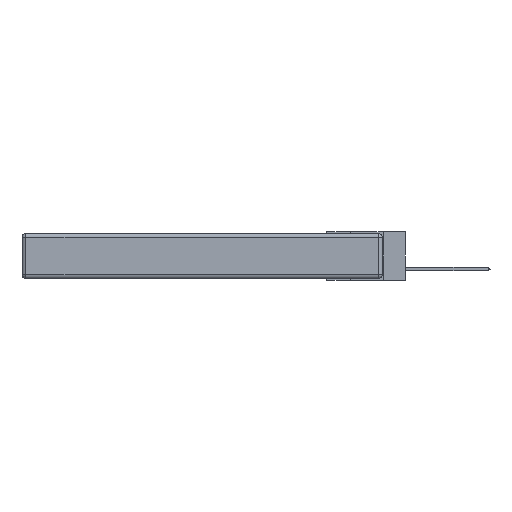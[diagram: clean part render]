
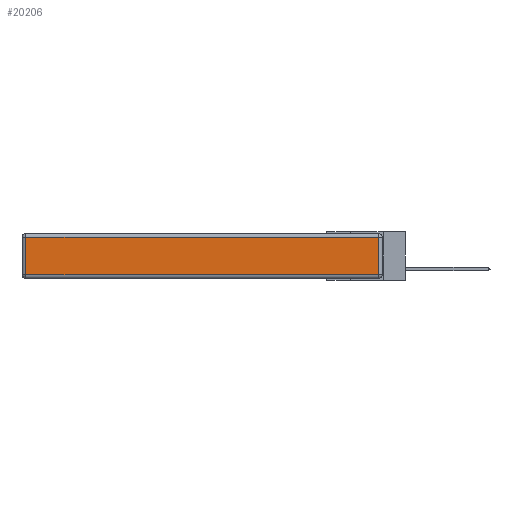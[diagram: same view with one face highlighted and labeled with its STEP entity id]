
A CAD part, left-side view. The second image highlights one B-rep face of the part: STEP entity #20206.
In plain terms, the highlighted planar face has unit normal (-1, 0, 0).
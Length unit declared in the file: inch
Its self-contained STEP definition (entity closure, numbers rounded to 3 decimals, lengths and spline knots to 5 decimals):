
#370 = VERTEX_POINT ( 'NONE', #17069 ) ;
#1235 = VECTOR ( 'NONE', #6113, 39.37008 ) ;
#2106 = VECTOR ( 'NONE', #9642, 39.37008 ) ;
#2582 = DIRECTION ( 'NONE',  ( 0., 0., -1. ) ) ;
#3070 = LINE ( 'NONE', #13655, #12551 ) ;
#6113 = DIRECTION ( 'NONE',  ( 0., 1., 0. ) ) ;
#6218 = EDGE_CURVE ( 'NONE', #370, #7089, #12154, .T. ) ;
#6316 = EDGE_CURVE ( 'NONE', #11339, #370, #19280, .T. ) ;
#6589 = ORIENTED_EDGE ( 'NONE', *, *, #10112, .T. ) ;
#7089 = VERTEX_POINT ( 'NONE', #19322 ) ;
#7811 = CARTESIAN_POINT ( 'NONE',  ( 0., 0.03, -0.343 ) ) ;
#8239 = VERTEX_POINT ( 'NONE', #21363 ) ;
#8573 = ORIENTED_EDGE ( 'NONE', *, *, #6218, .T. ) ;
#9642 = DIRECTION ( 'NONE',  ( 0., -1., 0. ) ) ;
#10112 = EDGE_CURVE ( 'NONE', #7089, #8239, #3070, .T. ) ;
#10745 = EDGE_CURVE ( 'NONE', #8239, #11339, #16156, .T. ) ;
#11339 = VERTEX_POINT ( 'NONE', #16797 ) ;
#11416 = EDGE_LOOP ( 'NONE', ( #15464, #17582, #8573, #6589 ) ) ;
#11490 = DIRECTION ( 'NONE',  ( 0., 0., 1. ) ) ;
#11632 = CARTESIAN_POINT ( 'NONE',  ( 0., 0., -0.313 ) ) ;
#12154 = LINE ( 'NONE', #18725, #1235 ) ;
#12551 = VECTOR ( 'NONE', #2582, 39.37008 ) ;
#13244 = AXIS2_PLACEMENT_3D ( 'NONE', #15725, #20925, #19308 ) ;
#13655 = CARTESIAN_POINT ( 'NONE',  ( 0., 2.72, -0.343 ) ) ;
#15464 = ORIENTED_EDGE ( 'NONE', *, *, #10745, .T. ) ;
#15725 = CARTESIAN_POINT ( 'NONE',  ( 0., 0., -0.343 ) ) ;
#16156 = LINE ( 'NONE', #11632, #2106 ) ;
#16785 = FACE_OUTER_BOUND ( 'NONE', #11416, .T. ) ;
#16797 = CARTESIAN_POINT ( 'NONE',  ( 0., 0.03, -0.313 ) ) ;
#17069 = CARTESIAN_POINT ( 'NONE',  ( 0., 0.03, -0.03 ) ) ;
#17582 = ORIENTED_EDGE ( 'NONE', *, *, #6316, .T. ) ;
#18725 = CARTESIAN_POINT ( 'NONE',  ( 0., 2.75, -0.03 ) ) ;
#19280 = LINE ( 'NONE', #7811, #23596 ) ;
#19308 = DIRECTION ( 'NONE',  ( 0., 0., 1. ) ) ;
#19322 = CARTESIAN_POINT ( 'NONE',  ( 0., 2.72, -0.03 ) ) ;
#20206 = ADVANCED_FACE ( 'NONE', ( #16785 ), #23076, .T. ) ;
#20925 = DIRECTION ( 'NONE',  ( -1., 0., 0. ) ) ;
#21363 = CARTESIAN_POINT ( 'NONE',  ( 0., 2.72, -0.313 ) ) ;
#23076 = PLANE ( 'NONE',  #13244 ) ;
#23596 = VECTOR ( 'NONE', #11490, 39.37008 ) ;
